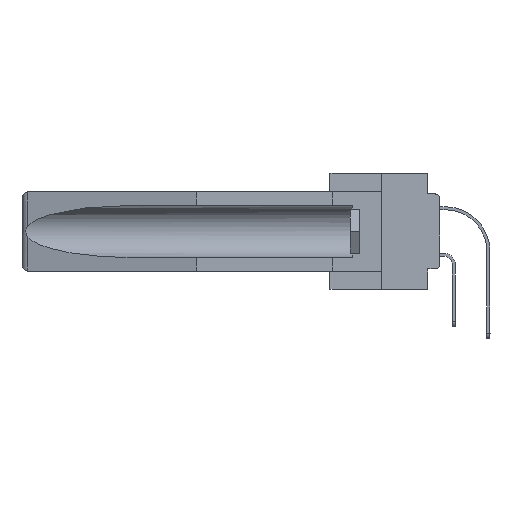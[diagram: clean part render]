
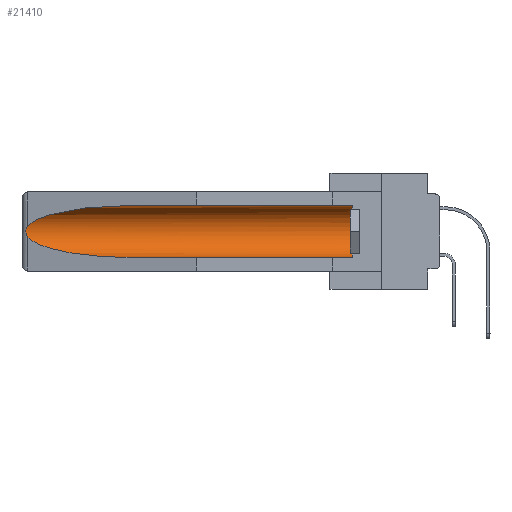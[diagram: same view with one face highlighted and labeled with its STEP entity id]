
A CAD part, left-side view. The second image highlights one B-rep face of the part: STEP entity #21410.
In plain terms, the highlighted cylindrical face has radius 2.857 mm (diameter 5.715 mm), a partial arc.
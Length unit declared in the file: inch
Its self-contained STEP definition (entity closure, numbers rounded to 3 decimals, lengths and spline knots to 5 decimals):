
#1527 = CARTESIAN_POINT ( 'NONE',  ( 0.2675, 1.53308, -0.17534 ) ) ;
#1610 = CARTESIAN_POINT ( 'NONE',  ( 0.155, 1.07973, -0.284 ) ) ;
#1701 =( BOUNDED_CURVE ( )  B_SPLINE_CURVE ( 3, ( #2359, #29346, #21338, #10705 ),
 .UNSPECIFIED., .F., .F. ) 
 B_SPLINE_CURVE_WITH_KNOTS ( ( 4, 4 ),
 ( 4.71239, 6.08839 ),
 .UNSPECIFIED. ) 
 CURVE ( )  GEOMETRIC_REPRESENTATION_ITEM ( )  RATIONAL_B_SPLINE_CURVE ( ( 1., 0.848, 0.848, 1. ) ) 
 REPRESENTATION_ITEM ( '' )  );
#1892 = ORIENTED_EDGE ( 'NONE', *, *, #5927, .F. ) ;
#2359 = CARTESIAN_POINT ( 'NONE',  ( 0.155, 1.07973, -0.059 ) ) ;
#2883 = EDGE_CURVE ( 'NONE', #30284, #3423, #18342, .T. ) ;
#3101 = CARTESIAN_POINT ( 'NONE',  ( 0.21114, 1.30732, -0.284 ) ) ;
#3423 = VERTEX_POINT ( 'NONE', #21247 ) ;
#3772 = VECTOR ( 'NONE', #28999, 39.37008 ) ;
#4122 = CARTESIAN_POINT ( 'NONE',  ( 0.2675, 1.53308, -0.16763 ) ) ;
#4799 = DIRECTION ( 'NONE',  ( 0., 0., 1. ) ) ;
#4987 = VECTOR ( 'NONE', #6624, 39.37008 ) ;
#5199 = VERTEX_POINT ( 'NONE', #1610 ) ;
#5443 = ORIENTED_EDGE ( 'NONE', *, *, #8357, .T. ) ;
#5861 = AXIS2_PLACEMENT_3D ( 'NONE', #19109, #14041, #21906 ) ;
#5927 = EDGE_CURVE ( 'NONE', #7832, #5199, #24595, .T. ) ;
#6291 = CARTESIAN_POINT ( 'NONE',  ( 0.155, -0.30754, -0.284 ) ) ;
#6624 = DIRECTION ( 'NONE',  ( 0., 1., 0. ) ) ;
#6719 = CARTESIAN_POINT ( 'NONE',  ( 0.2673, 1.5327, -0.16383 ) ) ;
#7455 = VERTEX_POINT ( 'NONE', #16527 ) ;
#7832 = VERTEX_POINT ( 'NONE', #15962 ) ;
#8357 = EDGE_CURVE ( 'NONE', #7455, #18403, #29998, .T. ) ;
#9491 = ORIENTED_EDGE ( 'NONE', *, *, #25562, .T. ) ;
#10705 = CARTESIAN_POINT ( 'NONE',  ( 0.26537, 1.52718, -0.14972 ) ) ;
#11766 = DIRECTION ( 'NONE',  ( 0., 1., 0. ) ) ;
#12120 = CARTESIAN_POINT ( 'NONE',  ( 0.2673, 1.53269, -0.17917 ) ) ;
#13804 = CARTESIAN_POINT ( 'NONE',  ( 0.155, 1.07973, -0.059 ) ) ;
#14041 = DIRECTION ( 'NONE',  ( 0., -1., 0. ) ) ;
#14365 = CARTESIAN_POINT ( 'NONE',  ( 0.155, -0.30754, -0.1715 ) ) ;
#15437 = ORIENTED_EDGE ( 'NONE', *, *, #2883, .T. ) ;
#15962 = CARTESIAN_POINT ( 'NONE',  ( 0.155, 0.126, -0.284 ) ) ;
#16485 = CARTESIAN_POINT ( 'NONE',  ( 0.155, 1.07973, -0.284 ) ) ;
#16527 = CARTESIAN_POINT ( 'NONE',  ( 0.155, 0.126, -0.059 ) ) ;
#18342 = B_SPLINE_CURVE_WITH_KNOTS ( 'NONE', 3,
 ( #25194, #19966, #30601, #6719, #4122, #1527, #12120, #22755, #20134, #30769 ),
 .UNSPECIFIED., .F., .F.,
 ( 4, 2, 2, 2, 4 ),
 ( 0., 0.00029, 0.00058, 0.00087, 0.00117 ),
 .UNSPECIFIED. ) ;
#18403 = VERTEX_POINT ( 'NONE', #13804 ) ;
#18785 = EDGE_LOOP ( 'NONE', ( #28800, #15437, #27035, #1892, #9491, #5443 ) ) ;
#19109 = CARTESIAN_POINT ( 'NONE',  ( 0.155, 0.126, -0.1715 ) ) ;
#19398 = CARTESIAN_POINT ( 'NONE',  ( 0.26537, 1.52718, -0.14972 ) ) ;
#19966 = CARTESIAN_POINT ( 'NONE',  ( 0.26597, 1.52961, -0.15275 ) ) ;
#20134 = CARTESIAN_POINT ( 'NONE',  ( 0.26597, 1.5296, -0.19026 ) ) ;
#21247 = CARTESIAN_POINT ( 'NONE',  ( 0.26537, 1.52718, -0.19328 ) ) ;
#21281 = AXIS2_PLACEMENT_3D ( 'NONE', #14365, #11766, #4799 ) ;
#21338 = CARTESIAN_POINT ( 'NONE',  ( 0.25451, 1.48313, -0.09465 ) ) ;
#21410 = ADVANCED_FACE ( 'NONE', ( #32857 ), #30250, .F. ) ;
#21906 = DIRECTION ( 'NONE',  ( 0., 0., 1. ) ) ;
#22755 = CARTESIAN_POINT ( 'NONE',  ( 0.26655, 1.53094, -0.18657 ) ) ;
#24160 = EDGE_CURVE ( 'NONE', #3423, #5199, #32819, .T. ) ;
#24595 = LINE ( 'NONE', #6291, #4987 ) ;
#25194 = CARTESIAN_POINT ( 'NONE',  ( 0.26537, 1.52718, -0.14972 ) ) ;
#25562 = EDGE_CURVE ( 'NONE', #7832, #7455, #30888, .T. ) ;
#25784 = EDGE_CURVE ( 'NONE', #18403, #30284, #1701, .T. ) ;
#27035 = ORIENTED_EDGE ( 'NONE', *, *, #24160, .T. ) ;
#27472 = CARTESIAN_POINT ( 'NONE',  ( 0.25451, 1.48313, -0.24835 ) ) ;
#28800 = ORIENTED_EDGE ( 'NONE', *, *, #25784, .T. ) ;
#28999 = DIRECTION ( 'NONE',  ( 0., 1., 0. ) ) ;
#29346 = CARTESIAN_POINT ( 'NONE',  ( 0.21114, 1.30732, -0.059 ) ) ;
#29998 = LINE ( 'NONE', #32133, #3772 ) ;
#30250 = CYLINDRICAL_SURFACE ( 'NONE', #21281, 0.1125 ) ;
#30284 = VERTEX_POINT ( 'NONE', #19398 ) ;
#30601 = CARTESIAN_POINT ( 'NONE',  ( 0.26654, 1.53092, -0.15636 ) ) ;
#30769 = CARTESIAN_POINT ( 'NONE',  ( 0.26537, 1.52718, -0.19328 ) ) ;
#30888 = CIRCLE ( 'NONE', #5861, 0.1125 ) ;
#32133 = CARTESIAN_POINT ( 'NONE',  ( 0.155, -0.30754, -0.059 ) ) ;
#32523 = CARTESIAN_POINT ( 'NONE',  ( 0.26537, 1.52718, -0.19328 ) ) ;
#32819 =( BOUNDED_CURVE ( )  B_SPLINE_CURVE ( 3, ( #32523, #27472, #3101, #16485 ),
 .UNSPECIFIED., .F., .F. ) 
 B_SPLINE_CURVE_WITH_KNOTS ( ( 4, 4 ),
 ( 0.1948, 1.5708 ),
 .UNSPECIFIED. ) 
 CURVE ( )  GEOMETRIC_REPRESENTATION_ITEM ( )  RATIONAL_B_SPLINE_CURVE ( ( 1., 0.848, 0.848, 1. ) ) 
 REPRESENTATION_ITEM ( '' )  );
#32857 = FACE_OUTER_BOUND ( 'NONE', #18785, .T. ) ;
